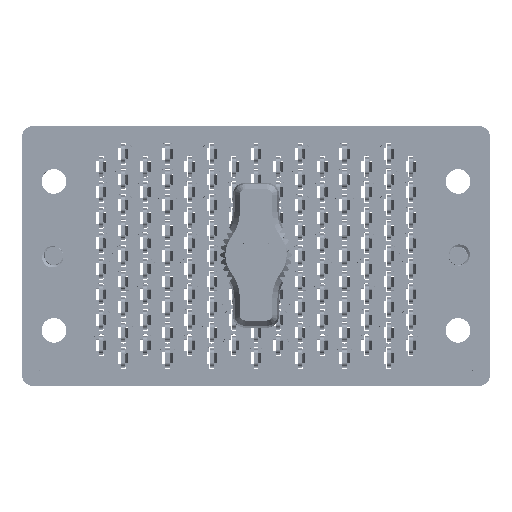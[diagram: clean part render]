
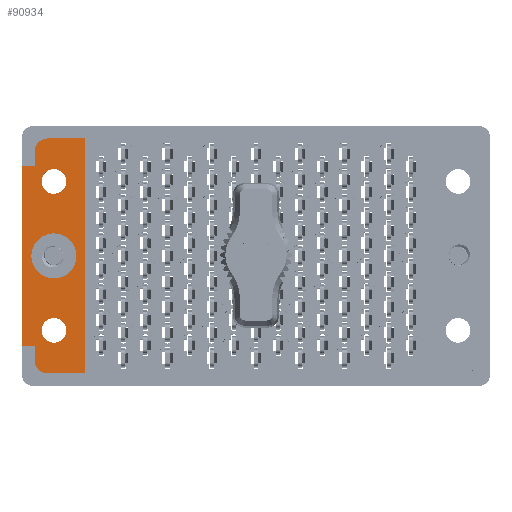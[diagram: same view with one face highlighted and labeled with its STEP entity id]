
A CAD part, top view. The second image highlights one B-rep face of the part: STEP entity #90934.
In plain terms, the highlighted planar face has unit normal (0, 0, 1).
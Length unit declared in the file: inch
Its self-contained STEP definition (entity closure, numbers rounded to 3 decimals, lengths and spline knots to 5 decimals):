
#1382 = VECTOR ( 'NONE', #38108, 39.37008 ) ;
#1569 = VERTEX_POINT ( 'NONE', #31288 ) ;
#1663 = DIRECTION ( 'NONE',  ( 1., 0., 0. ) ) ;
#2108 = DIRECTION ( 'NONE',  ( 1., 0., 0. ) ) ;
#4455 = CARTESIAN_POINT ( 'NONE',  ( -1.1875, 0., -0.117 ) ) ;
#4687 = EDGE_CURVE ( 'NONE', #37759, #35082, #116131, .T. ) ;
#6320 = AXIS2_PLACEMENT_3D ( 'NONE', #53620, #63841, #45708 ) ;
#6366 = EDGE_CURVE ( 'NONE', #112839, #112275, #22714, .T. ) ;
#6498 = CARTESIAN_POINT ( 'NONE',  ( -1.1875, -0.4375, -0.117 ) ) ;
#7439 = CIRCLE ( 'NONE', #6320, 0.075 ) ;
#7509 = AXIS2_PLACEMENT_3D ( 'NONE', #110775, #20930, #1663 ) ;
#7909 = ORIENTED_EDGE ( 'NONE', *, *, #32633, .T. ) ;
#8417 = CARTESIAN_POINT ( 'NONE',  ( -1.3, 0.5285, -0.117 ) ) ;
#10651 = CARTESIAN_POINT ( 'NONE',  ( -1.375, 0.7625, -0.117 ) ) ;
#10928 = LINE ( 'NONE', #64948, #116611 ) ;
#12552 = EDGE_LOOP ( 'NONE', ( #37001, #93915 ) ) ;
#12571 = CARTESIAN_POINT ( 'NONE',  ( -1.1875, 0.4375, -0.117 ) ) ;
#12961 = DIRECTION ( 'NONE',  ( 0., 0., 1. ) ) ;
#15567 = DIRECTION ( 'NONE',  ( 1., 0., 0. ) ) ;
#17900 = ORIENTED_EDGE ( 'NONE', *, *, #32993, .F. ) ;
#18600 = CARTESIAN_POINT ( 'NONE',  ( -1.375, 0.5285, -0.117 ) ) ;
#18676 = ORIENTED_EDGE ( 'NONE', *, *, #88240, .T. ) ;
#18913 = DIRECTION ( 'NONE',  ( 0., -1., 0. ) ) ;
#19306 = CARTESIAN_POINT ( 'NONE',  ( -1.375, -0.5285, -0.117 ) ) ;
#19579 = DIRECTION ( 'NONE',  ( 1., 0., 0. ) ) ;
#20930 = DIRECTION ( 'NONE',  ( 0., 0., 1. ) ) ;
#21061 = AXIS2_PLACEMENT_3D ( 'NONE', #73168, #64522, #19579 ) ;
#21203 = DIRECTION ( 'NONE',  ( 1., 0., 0. ) ) ;
#22132 = CARTESIAN_POINT ( 'NONE',  ( -1.3, -0.5285, -0.117 ) ) ;
#22152 = DIRECTION ( 'NONE',  ( -1., 0., 0. ) ) ;
#22244 = ORIENTED_EDGE ( 'NONE', *, *, #94721, .T. ) ;
#22714 = CIRCLE ( 'NONE', #69910, 0.0725 ) ;
#24619 = ORIENTED_EDGE ( 'NONE', *, *, #25426, .F. ) ;
#24728 = AXIS2_PLACEMENT_3D ( 'NONE', #110305, #74493, #38644 ) ;
#25052 = EDGE_CURVE ( 'NONE', #112275, #112839, #35175, .T. ) ;
#25313 = CARTESIAN_POINT ( 'NONE',  ( -1.005, 0.69, -0.117 ) ) ;
#25426 = EDGE_CURVE ( 'NONE', #114933, #26826, #73378, .T. ) ;
#25571 = ORIENTED_EDGE ( 'NONE', *, *, #6366, .F. ) ;
#26512 = VERTEX_POINT ( 'NONE', #32013 ) ;
#26826 = VERTEX_POINT ( 'NONE', #43411 ) ;
#26944 = EDGE_CURVE ( 'NONE', #38975, #1569, #94462, .T. ) ;
#28397 = AXIS2_PLACEMENT_3D ( 'NONE', #6498, #43156, #15567 ) ;
#28623 = CARTESIAN_POINT ( 'NONE',  ( 0., 0.5285, -0.117 ) ) ;
#28694 = ORIENTED_EDGE ( 'NONE', *, *, #4687, .T. ) ;
#28883 = EDGE_CURVE ( 'NONE', #114933, #107322, #92687, .T. ) ;
#29074 = DIRECTION ( 'NONE',  ( 0., -1., 0. ) ) ;
#30069 = ORIENTED_EDGE ( 'NONE', *, *, #38693, .T. ) ;
#31288 = CARTESIAN_POINT ( 'NONE',  ( -1.115, 0.4375, -0.117 ) ) ;
#31431 = EDGE_LOOP ( 'NONE', ( #56388, #17900 ) ) ;
#31629 = DIRECTION ( 'NONE',  ( 0., 0., 1. ) ) ;
#32013 = CARTESIAN_POINT ( 'NONE',  ( -1.055, 0., -0.117 ) ) ;
#32633 = EDGE_CURVE ( 'NONE', #113796, #26826, #7439, .T. ) ;
#32993 = EDGE_CURVE ( 'NONE', #1569, #38975, #87146, .T. ) ;
#34570 = VERTEX_POINT ( 'NONE', #22132 ) ;
#35082 = VERTEX_POINT ( 'NONE', #19306 ) ;
#35175 = CIRCLE ( 'NONE', #28397, 0.0725 ) ;
#35986 = DIRECTION ( 'NONE',  ( 0., 0., 1. ) ) ;
#37001 = ORIENTED_EDGE ( 'NONE', *, *, #69496, .F. ) ;
#37135 = EDGE_CURVE ( 'NONE', #55178, #103432, #91629, .T. ) ;
#37759 = VERTEX_POINT ( 'NONE', #18600 ) ;
#38108 = DIRECTION ( 'NONE',  ( -1., 0., 0. ) ) ;
#38644 = DIRECTION ( 'NONE',  ( 1., 0., 0. ) ) ;
#38693 = EDGE_CURVE ( 'NONE', #107322, #55178, #43391, .T. ) ;
#38975 = VERTEX_POINT ( 'NONE', #46245 ) ;
#43156 = DIRECTION ( 'NONE',  ( 0., 0., 1. ) ) ;
#43391 = LINE ( 'NONE', #48005, #101082 ) ;
#43411 = CARTESIAN_POINT ( 'NONE',  ( -1.225, -0.69, -0.117 ) ) ;
#43622 = ORIENTED_EDGE ( 'NONE', *, *, #89765, .T. ) ;
#44775 = VECTOR ( 'NONE', #114568, 39.37008 ) ;
#44872 = DIRECTION ( 'NONE',  ( 0., -1., 0. ) ) ;
#45708 = DIRECTION ( 'NONE',  ( 1., 0., 0. ) ) ;
#46245 = CARTESIAN_POINT ( 'NONE',  ( -1.26, 0.4375, -0.117 ) ) ;
#46964 = PLANE ( 'NONE',  #7509 ) ;
#47106 = CARTESIAN_POINT ( 'NONE',  ( 0., -0.5285, -0.117 ) ) ;
#48005 = CARTESIAN_POINT ( 'NONE',  ( 0., 0.69, -0.117 ) ) ;
#48402 = DIRECTION ( 'NONE',  ( -1., 0., 0. ) ) ;
#48641 = DIRECTION ( 'NONE',  ( 1., 0., 0. ) ) ;
#50145 = FACE_BOUND ( 'NONE', #103043, .T. ) ;
#51154 = CARTESIAN_POINT ( 'NONE',  ( -1.005, 0.7625, -0.117 ) ) ;
#52475 = ORIENTED_EDGE ( 'NONE', *, *, #25052, .F. ) ;
#53620 = CARTESIAN_POINT ( 'NONE',  ( -1.225, -0.615, -0.117 ) ) ;
#55178 = VERTEX_POINT ( 'NONE', #74434 ) ;
#55795 = AXIS2_PLACEMENT_3D ( 'NONE', #4455, #31629, #48641 ) ;
#56123 = ORIENTED_EDGE ( 'NONE', *, *, #90361, .F. ) ;
#56388 = ORIENTED_EDGE ( 'NONE', *, *, #26944, .F. ) ;
#57757 = VECTOR ( 'NONE', #44872, 39.37008 ) ;
#63841 = DIRECTION ( 'NONE',  ( 0., 0., 1. ) ) ;
#64070 = EDGE_LOOP ( 'NONE', ( #30069, #99158, #18676, #22244, #28694, #56123, #43622, #7909, #24619, #67440 ) ) ;
#64522 = DIRECTION ( 'NONE',  ( 0., 0., 1. ) ) ;
#64948 = CARTESIAN_POINT ( 'NONE',  ( -1.3, 0., -0.117 ) ) ;
#67440 = ORIENTED_EDGE ( 'NONE', *, *, #28883, .T. ) ;
#68428 = FACE_BOUND ( 'NONE', #31431, .T. ) ;
#69496 = EDGE_CURVE ( 'NONE', #26512, #89507, #105781, .T. ) ;
#69910 = AXIS2_PLACEMENT_3D ( 'NONE', #89944, #35986, #2108 ) ;
#71300 = CARTESIAN_POINT ( 'NONE',  ( -1.3, 0.615, -0.117 ) ) ;
#73168 = CARTESIAN_POINT ( 'NONE',  ( -1.1875, 0., -0.117 ) ) ;
#73378 = LINE ( 'NONE', #103260, #93701 ) ;
#74127 = FACE_OUTER_BOUND ( 'NONE', #64070, .T. ) ;
#74434 = CARTESIAN_POINT ( 'NONE',  ( -1.225, 0.69, -0.117 ) ) ;
#74493 = DIRECTION ( 'NONE',  ( 0., 0., 1. ) ) ;
#77471 = LINE ( 'NONE', #28623, #1382 ) ;
#78303 = FACE_BOUND ( 'NONE', #12552, .T. ) ;
#81713 = LINE ( 'NONE', #89766, #57757 ) ;
#82698 = VERTEX_POINT ( 'NONE', #8417 ) ;
#86881 = LINE ( 'NONE', #47106, #109351 ) ;
#87146 = CIRCLE ( 'NONE', #111273, 0.0725 ) ;
#88240 = EDGE_CURVE ( 'NONE', #103432, #82698, #81713, .T. ) ;
#89507 = VERTEX_POINT ( 'NONE', #114227 ) ;
#89765 = EDGE_CURVE ( 'NONE', #34570, #113796, #10928, .T. ) ;
#89766 = CARTESIAN_POINT ( 'NONE',  ( -1.3, 0., -0.117 ) ) ;
#89944 = CARTESIAN_POINT ( 'NONE',  ( -1.1875, -0.4375, -0.117 ) ) ;
#90361 = EDGE_CURVE ( 'NONE', #34570, #35082, #86881, .T. ) ;
#90934 = ADVANCED_FACE ( 'NONE', ( #68428, #50145, #78303, #74127 ), #46964, .T. ) ;
#91174 = CARTESIAN_POINT ( 'NONE',  ( -1.3, -0.615, -0.117 ) ) ;
#91221 = DIRECTION ( 'NONE',  ( -1., 0., 0. ) ) ;
#91301 = CARTESIAN_POINT ( 'NONE',  ( -1.225, 0.615, -0.117 ) ) ;
#91629 = CIRCLE ( 'NONE', #93454, 0.075 ) ;
#92146 = VECTOR ( 'NONE', #18913, 39.37008 ) ;
#92687 = LINE ( 'NONE', #51154, #44775 ) ;
#93360 = CARTESIAN_POINT ( 'NONE',  ( -1.005, -0.69, -0.117 ) ) ;
#93454 = AXIS2_PLACEMENT_3D ( 'NONE', #91301, #110606, #110202 ) ;
#93701 = VECTOR ( 'NONE', #22152, 39.37008 ) ;
#93915 = ORIENTED_EDGE ( 'NONE', *, *, #97544, .F. ) ;
#94462 = CIRCLE ( 'NONE', #24728, 0.0725 ) ;
#94721 = EDGE_CURVE ( 'NONE', #82698, #37759, #77471, .T. ) ;
#97544 = EDGE_CURVE ( 'NONE', #89507, #26512, #104890, .T. ) ;
#99158 = ORIENTED_EDGE ( 'NONE', *, *, #37135, .T. ) ;
#101082 = VECTOR ( 'NONE', #48402, 39.37008 ) ;
#101200 = CARTESIAN_POINT ( 'NONE',  ( -1.115, -0.4375, -0.117 ) ) ;
#103043 = EDGE_LOOP ( 'NONE', ( #25571, #52475 ) ) ;
#103260 = CARTESIAN_POINT ( 'NONE',  ( 0., -0.69, -0.117 ) ) ;
#103432 = VERTEX_POINT ( 'NONE', #71300 ) ;
#104890 = CIRCLE ( 'NONE', #21061, 0.1325 ) ;
#105781 = CIRCLE ( 'NONE', #55795, 0.1325 ) ;
#106308 = CARTESIAN_POINT ( 'NONE',  ( -1.26, -0.4375, -0.117 ) ) ;
#107322 = VERTEX_POINT ( 'NONE', #25313 ) ;
#109351 = VECTOR ( 'NONE', #91221, 39.37008 ) ;
#110202 = DIRECTION ( 'NONE',  ( 1., 0., 0. ) ) ;
#110305 = CARTESIAN_POINT ( 'NONE',  ( -1.1875, 0.4375, -0.117 ) ) ;
#110606 = DIRECTION ( 'NONE',  ( 0., 0., 1. ) ) ;
#110775 = CARTESIAN_POINT ( 'NONE',  ( -1.375, -0.7625, -0.117 ) ) ;
#111273 = AXIS2_PLACEMENT_3D ( 'NONE', #12571, #12961, #21203 ) ;
#112275 = VERTEX_POINT ( 'NONE', #101200 ) ;
#112839 = VERTEX_POINT ( 'NONE', #106308 ) ;
#113796 = VERTEX_POINT ( 'NONE', #91174 ) ;
#114227 = CARTESIAN_POINT ( 'NONE',  ( -1.32, 0., -0.117 ) ) ;
#114568 = DIRECTION ( 'NONE',  ( 0., 1., 0. ) ) ;
#114933 = VERTEX_POINT ( 'NONE', #93360 ) ;
#116131 = LINE ( 'NONE', #10651, #92146 ) ;
#116611 = VECTOR ( 'NONE', #29074, 39.37008 ) ;
